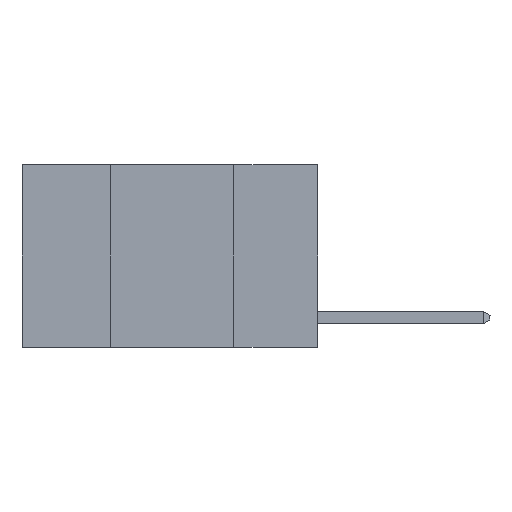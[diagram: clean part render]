
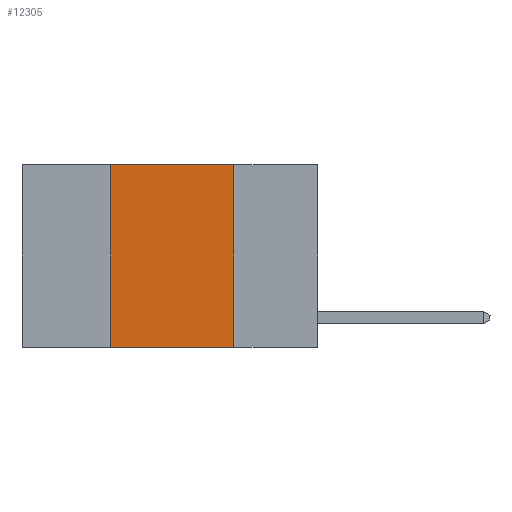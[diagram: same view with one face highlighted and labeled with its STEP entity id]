
A CAD part, left-side view. The second image highlights one B-rep face of the part: STEP entity #12305.
In plain terms, the highlighted planar face has unit normal (-1, 0, 0).
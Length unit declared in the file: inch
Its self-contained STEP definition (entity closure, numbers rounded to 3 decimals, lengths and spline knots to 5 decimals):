
#112 = CARTESIAN_POINT ( 'NONE',  ( 0., 0.42, 0. ) ) ;
#532 = CARTESIAN_POINT ( 'NONE',  ( 0., 0.6, 0. ) ) ;
#1526 = EDGE_CURVE ( 'NONE', #15296, #18511, #8877, .T. ) ;
#2063 = CARTESIAN_POINT ( 'NONE',  ( 0., 0.17, -0.37 ) ) ;
#2898 = FACE_OUTER_BOUND ( 'NONE', #6895, .T. ) ;
#3053 = DIRECTION ( 'NONE',  ( 0., 0., 1. ) ) ;
#3087 = VECTOR ( 'NONE', #3053, 39.37008 ) ;
#3331 = ORIENTED_EDGE ( 'NONE', *, *, #11368, .F. ) ;
#3953 = VERTEX_POINT ( 'NONE', #18300 ) ;
#4173 = CARTESIAN_POINT ( 'NONE',  ( 0., 0.6, -0.37 ) ) ;
#4301 = DIRECTION ( 'NONE',  ( 0., 0., -1. ) ) ;
#4626 = EDGE_CURVE ( 'NONE', #3953, #18511, #16463, .T. ) ;
#4719 = CARTESIAN_POINT ( 'NONE',  ( 0., 0.17, 0. ) ) ;
#6534 = VECTOR ( 'NONE', #4301, 39.37008 ) ;
#6895 = EDGE_LOOP ( 'NONE', ( #18265, #3331, #12074, #13836 ) ) ;
#7505 = VECTOR ( 'NONE', #15142, 39.37008 ) ;
#8625 = EDGE_CURVE ( 'NONE', #3953, #16712, #11973, .T. ) ;
#8856 = PLANE ( 'NONE',  #10057 ) ;
#8877 = LINE ( 'NONE', #11654, #6534 ) ;
#9871 = VECTOR ( 'NONE', #10142, 39.37008 ) ;
#10057 = AXIS2_PLACEMENT_3D ( 'NONE', #532, #12586, #13752 ) ;
#10142 = DIRECTION ( 'NONE',  ( 0., -1., 0. ) ) ;
#11368 = EDGE_CURVE ( 'NONE', #16712, #15296, #14706, .T. ) ;
#11654 = CARTESIAN_POINT ( 'NONE',  ( 0., 0.17, 0. ) ) ;
#11973 = LINE ( 'NONE', #16447, #3087 ) ;
#12074 = ORIENTED_EDGE ( 'NONE', *, *, #8625, .F. ) ;
#12141 = CARTESIAN_POINT ( 'NONE',  ( 0., 0.6, 0. ) ) ;
#12305 = ADVANCED_FACE ( 'NONE', ( #2898 ), #8856, .F. ) ;
#12586 = DIRECTION ( 'NONE',  ( 1., 0., 0. ) ) ;
#13752 = DIRECTION ( 'NONE',  ( 0., 0., -1. ) ) ;
#13836 = ORIENTED_EDGE ( 'NONE', *, *, #4626, .T. ) ;
#14706 = LINE ( 'NONE', #12141, #7505 ) ;
#15142 = DIRECTION ( 'NONE',  ( 0., -1., 0. ) ) ;
#15296 = VERTEX_POINT ( 'NONE', #4719 ) ;
#16447 = CARTESIAN_POINT ( 'NONE',  ( 0., 0.42, 0. ) ) ;
#16463 = LINE ( 'NONE', #4173, #9871 ) ;
#16712 = VERTEX_POINT ( 'NONE', #112 ) ;
#18265 = ORIENTED_EDGE ( 'NONE', *, *, #1526, .F. ) ;
#18300 = CARTESIAN_POINT ( 'NONE',  ( 0., 0.42, -0.37 ) ) ;
#18511 = VERTEX_POINT ( 'NONE', #2063 ) ;
